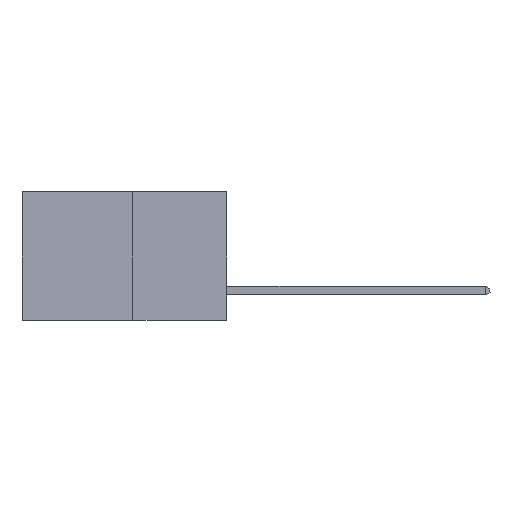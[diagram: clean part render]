
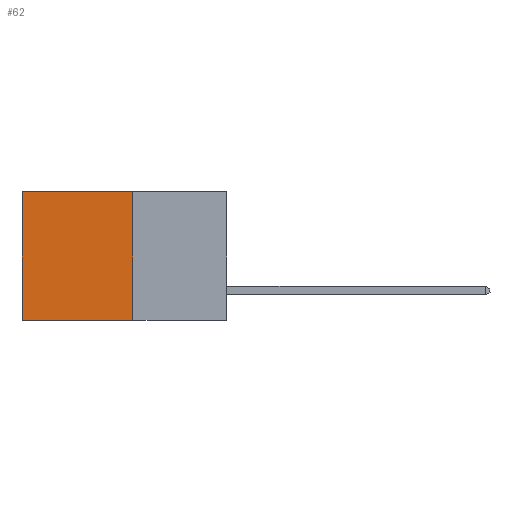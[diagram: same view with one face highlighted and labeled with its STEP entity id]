
A CAD part, left-side view. The second image highlights one B-rep face of the part: STEP entity #62.
In plain terms, the highlighted planar face has unit normal (-1, 0, 0).
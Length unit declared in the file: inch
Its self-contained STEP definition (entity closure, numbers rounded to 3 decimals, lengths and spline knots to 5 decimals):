
#30 = ORIENTED_EDGE ( 'NONE', *, *, #727, .F. ) ;
#62 = ADVANCED_FACE ( 'NONE', ( #2562 ), #1117, .F. ) ;
#73 = EDGE_CURVE ( 'NONE', #5910, #10003, #10205, .T. ) ;
#631 = LINE ( 'NONE', #2888, #10609 ) ;
#727 = EDGE_CURVE ( 'NONE', #10288, #5910, #631, .T. ) ;
#1117 = PLANE ( 'NONE',  #6526 ) ;
#1284 = ORIENTED_EDGE ( 'NONE', *, *, #11924, .T. ) ;
#2234 = DIRECTION ( 'NONE',  ( 0., 1., 0. ) ) ;
#2562 = FACE_OUTER_BOUND ( 'NONE', #3412, .T. ) ;
#2888 = CARTESIAN_POINT ( 'NONE',  ( 0.277, 0.27, -0.37 ) ) ;
#3412 = EDGE_LOOP ( 'NONE', ( #6052, #11538, #30, #1284 ) ) ;
#3532 = CARTESIAN_POINT ( 'NONE',  ( 0.277, 0.27, -0.37 ) ) ;
#3579 = DIRECTION ( 'NONE',  ( 0., 1., 0. ) ) ;
#4855 = VECTOR ( 'NONE', #2234, 39.37008 ) ;
#5253 = LINE ( 'NONE', #8790, #5583 ) ;
#5510 = DIRECTION ( 'NONE',  ( 0., 0., -1. ) ) ;
#5552 = CARTESIAN_POINT ( 'NONE',  ( 0.277, 0.27, 0. ) ) ;
#5583 = VECTOR ( 'NONE', #12371, 39.37008 ) ;
#5615 = VERTEX_POINT ( 'NONE', #8742 ) ;
#5681 = VECTOR ( 'NONE', #3579, 39.37008 ) ;
#5910 = VERTEX_POINT ( 'NONE', #9351 ) ;
#6052 = ORIENTED_EDGE ( 'NONE', *, *, #9334, .T. ) ;
#6526 = AXIS2_PLACEMENT_3D ( 'NONE', #3532, #11986, #8636 ) ;
#7893 = CARTESIAN_POINT ( 'NONE',  ( 0.277, 0.59, -0.37 ) ) ;
#8545 = LINE ( 'NONE', #5552, #5681 ) ;
#8636 = DIRECTION ( 'NONE',  ( 0., 0., -1. ) ) ;
#8742 = CARTESIAN_POINT ( 'NONE',  ( 0.277, 0.59, 0. ) ) ;
#8790 = CARTESIAN_POINT ( 'NONE',  ( 0.277, 0.59, -0.37 ) ) ;
#9334 = EDGE_CURVE ( 'NONE', #5615, #10003, #5253, .T. ) ;
#9351 = CARTESIAN_POINT ( 'NONE',  ( 0.277, 0.27, -0.37 ) ) ;
#9923 = CARTESIAN_POINT ( 'NONE',  ( 0.277, 0.27, -0.37 ) ) ;
#10003 = VERTEX_POINT ( 'NONE', #7893 ) ;
#10205 = LINE ( 'NONE', #9923, #4855 ) ;
#10288 = VERTEX_POINT ( 'NONE', #11841 ) ;
#10609 = VECTOR ( 'NONE', #5510, 39.37008 ) ;
#11538 = ORIENTED_EDGE ( 'NONE', *, *, #73, .F. ) ;
#11841 = CARTESIAN_POINT ( 'NONE',  ( 0.277, 0.27, 0. ) ) ;
#11924 = EDGE_CURVE ( 'NONE', #10288, #5615, #8545, .T. ) ;
#11986 = DIRECTION ( 'NONE',  ( 1., 0., 0. ) ) ;
#12371 = DIRECTION ( 'NONE',  ( 0., 0., -1. ) ) ;
